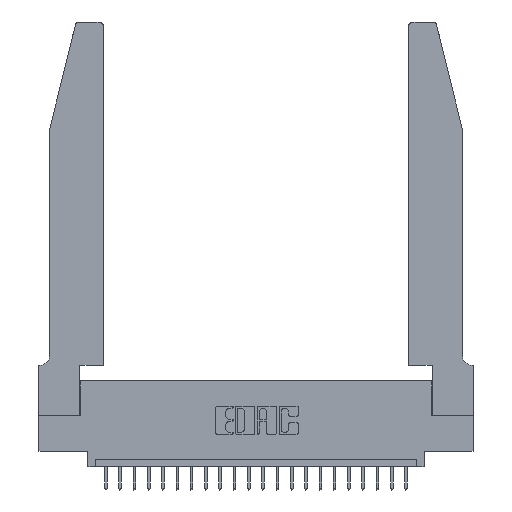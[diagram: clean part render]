
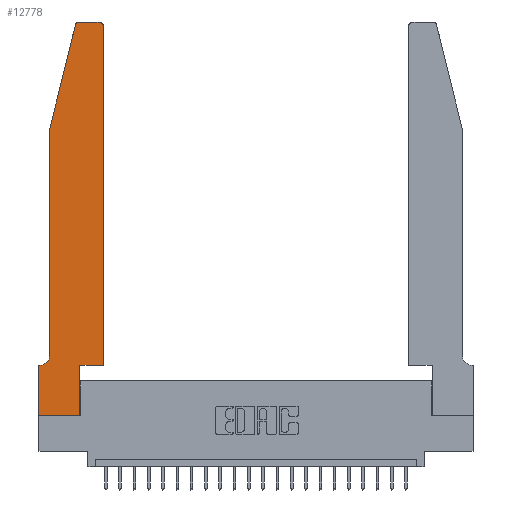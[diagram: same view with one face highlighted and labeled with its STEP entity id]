
A CAD part, top view. The second image highlights one B-rep face of the part: STEP entity #12778.
In plain terms, the highlighted planar face has unit normal (0, 0, 1).
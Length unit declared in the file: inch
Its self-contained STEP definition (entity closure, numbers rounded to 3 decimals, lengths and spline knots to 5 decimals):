
#12 = VERTEX_POINT ( 'NONE', #21400 ) ;
#245 = EDGE_CURVE ( 'NONE', #12, #11138, #21947, .T. ) ;
#420 = ORIENTED_EDGE ( 'NONE', *, *, #14623, .T. ) ;
#644 = DIRECTION ( 'NONE',  ( 1., 0., 0. ) ) ;
#722 = CARTESIAN_POINT ( 'NONE',  ( 0.4505, 0.35, 0.37 ) ) ;
#818 = VERTEX_POINT ( 'NONE', #722 ) ;
#968 = CARTESIAN_POINT ( 'NONE',  ( 0.0055, 0.35, 0.37 ) ) ;
#1003 = CARTESIAN_POINT ( 'NONE',  ( 0., 0.35, 0.37 ) ) ;
#1367 = LINE ( 'NONE', #20364, #1975 ) ;
#1441 = CARTESIAN_POINT ( 'NONE',  ( 0.4205, 2.72, 0.37 ) ) ;
#1541 = DIRECTION ( 'NONE',  ( 0., 0., -1. ) ) ;
#1650 = VERTEX_POINT ( 'NONE', #11311 ) ;
#1730 = VERTEX_POINT ( 'NONE', #23670 ) ;
#1876 = CARTESIAN_POINT ( 'NONE',  ( 0.2605, 2.75, 0.37 ) ) ;
#1975 = VECTOR ( 'NONE', #12963, 39.37008 ) ;
#2548 = ORIENTED_EDGE ( 'NONE', *, *, #4181, .T. ) ;
#2737 = CIRCLE ( 'NONE', #22688, 0.07 ) ;
#3608 = ORIENTED_EDGE ( 'NONE', *, *, #23975, .T. ) ;
#3681 = AXIS2_PLACEMENT_3D ( 'NONE', #12001, #17475, #15789 ) ;
#3734 = ORIENTED_EDGE ( 'NONE', *, *, #11519, .T. ) ;
#4095 = CIRCLE ( 'NONE', #3681, 0.03 ) ;
#4103 = VERTEX_POINT ( 'NONE', #8021 ) ;
#4181 = EDGE_CURVE ( 'NONE', #1730, #15587, #2737, .T. ) ;
#4785 = LINE ( 'NONE', #19580, #16541 ) ;
#5365 = VERTEX_POINT ( 'NONE', #7875 ) ;
#5584 = CARTESIAN_POINT ( 'NONE',  ( 0.4205, 2.75, 0.37 ) ) ;
#5873 = ORIENTED_EDGE ( 'NONE', *, *, #245, .T. ) ;
#5895 = EDGE_CURVE ( 'NONE', #5365, #20398, #1367, .T. ) ;
#6789 = EDGE_CURVE ( 'NONE', #20398, #1730, #19794, .T. ) ;
#7076 = DIRECTION ( 'NONE',  ( 1., 0., 0. ) ) ;
#7831 = EDGE_CURVE ( 'NONE', #15587, #19363, #4785, .T. ) ;
#7875 = CARTESIAN_POINT ( 'NONE',  ( 0.25487, 2.72718, 0.37 ) ) ;
#8021 = CARTESIAN_POINT ( 'NONE',  ( 0.2865, 0.35, 0.37 ) ) ;
#8172 = CARTESIAN_POINT ( 'NONE',  ( 0.4505, 0.35, 0.37 ) ) ;
#8364 = VECTOR ( 'NONE', #12646, 39.37008 ) ;
#8563 = CARTESIAN_POINT ( 'NONE',  ( 0.2865, 0., 0.37 ) ) ;
#8788 = ORIENTED_EDGE ( 'NONE', *, *, #6789, .T. ) ;
#8869 = VERTEX_POINT ( 'NONE', #21724 ) ;
#9479 = DIRECTION ( 'NONE',  ( 0., -1., 0. ) ) ;
#10090 = LINE ( 'NONE', #8172, #22071 ) ;
#10218 = LINE ( 'NONE', #1876, #18743 ) ;
#10506 = VECTOR ( 'NONE', #644, 39.37008 ) ;
#10783 = LINE ( 'NONE', #23120, #10506 ) ;
#10952 = DIRECTION ( 'NONE',  ( 0., 0., 1. ) ) ;
#11138 = VERTEX_POINT ( 'NONE', #8563 ) ;
#11145 = DIRECTION ( 'NONE',  ( -1., 0., 0. ) ) ;
#11148 = CARTESIAN_POINT ( 'NONE',  ( 0., 0., 0.37 ) ) ;
#11269 = DIRECTION ( 'NONE',  ( 1., 0., 0. ) ) ;
#11300 = DIRECTION ( 'NONE',  ( -1., 0., 0. ) ) ;
#11311 = CARTESIAN_POINT ( 'NONE',  ( 0.4505, 2.72, 0.37 ) ) ;
#11321 = AXIS2_PLACEMENT_3D ( 'NONE', #15298, #22427, #11269 ) ;
#11519 = EDGE_CURVE ( 'NONE', #16461, #8869, #10218, .T. ) ;
#11669 = EDGE_CURVE ( 'NONE', #4103, #818, #10783, .T. ) ;
#11670 = LINE ( 'NONE', #11148, #21845 ) ;
#12001 = CARTESIAN_POINT ( 'NONE',  ( 0.284, 2.72, 0.37 ) ) ;
#12327 = DIRECTION ( 'NONE',  ( -1., 0., 0. ) ) ;
#12646 = DIRECTION ( 'NONE',  ( 0., -1., 0. ) ) ;
#12778 = ADVANCED_FACE ( 'NONE', ( #16432 ), #17165, .T. ) ;
#12876 = CARTESIAN_POINT ( 'NONE',  ( 0., 0., 0.37 ) ) ;
#12921 = VECTOR ( 'NONE', #22213, 39.37008 ) ;
#12963 = DIRECTION ( 'NONE',  ( -0.239, -0.971, 0. ) ) ;
#14623 = EDGE_CURVE ( 'NONE', #19363, #12, #11670, .T. ) ;
#14729 = ORIENTED_EDGE ( 'NONE', *, *, #11669, .T. ) ;
#15298 = CARTESIAN_POINT ( 'NONE',  ( 0., 0.35, 0.37 ) ) ;
#15587 = VERTEX_POINT ( 'NONE', #968 ) ;
#15789 = DIRECTION ( 'NONE',  ( 1., 0., 0. ) ) ;
#15840 = DIRECTION ( 'NONE',  ( 0., 1., 0. ) ) ;
#16432 = FACE_OUTER_BOUND ( 'NONE', #24192, .T. ) ;
#16461 = VERTEX_POINT ( 'NONE', #5584 ) ;
#16541 = VECTOR ( 'NONE', #12327, 39.37008 ) ;
#16726 = CARTESIAN_POINT ( 'NONE',  ( 0.0055, 0.42, 0.37 ) ) ;
#17019 = EDGE_CURVE ( 'NONE', #818, #1650, #10090, .T. ) ;
#17165 = PLANE ( 'NONE',  #11321 ) ;
#17475 = DIRECTION ( 'NONE',  ( 0., 0., 1. ) ) ;
#17480 = ORIENTED_EDGE ( 'NONE', *, *, #5895, .T. ) ;
#17497 = ORIENTED_EDGE ( 'NONE', *, *, #19230, .T. ) ;
#18743 = VECTOR ( 'NONE', #11300, 39.37008 ) ;
#19230 = EDGE_CURVE ( 'NONE', #8869, #5365, #4095, .T. ) ;
#19363 = VERTEX_POINT ( 'NONE', #1003 ) ;
#19567 = ORIENTED_EDGE ( 'NONE', *, *, #17019, .T. ) ;
#19580 = CARTESIAN_POINT ( 'NONE',  ( 0.0755, 0.35, 0.37 ) ) ;
#19794 = LINE ( 'NONE', #21831, #8364 ) ;
#20082 = CARTESIAN_POINT ( 'NONE',  ( 0.2865, 0.35, 0.37 ) ) ;
#20364 = CARTESIAN_POINT ( 'NONE',  ( 0.0755, 2., 0.37 ) ) ;
#20398 = VERTEX_POINT ( 'NONE', #22776 ) ;
#20496 = ORIENTED_EDGE ( 'NONE', *, *, #7831, .T. ) ;
#20735 = EDGE_CURVE ( 'NONE', #11138, #4103, #23606, .T. ) ;
#21400 = CARTESIAN_POINT ( 'NONE',  ( 0., 0., 0.37 ) ) ;
#21574 = VECTOR ( 'NONE', #23569, 39.37008 ) ;
#21724 = CARTESIAN_POINT ( 'NONE',  ( 0.284, 2.75, 0.37 ) ) ;
#21831 = CARTESIAN_POINT ( 'NONE',  ( 0.0755, 2., 0.37 ) ) ;
#21845 = VECTOR ( 'NONE', #9479, 39.37008 ) ;
#21947 = LINE ( 'NONE', #12876, #12921 ) ;
#21982 = ORIENTED_EDGE ( 'NONE', *, *, #20735, .T. ) ;
#22071 = VECTOR ( 'NONE', #15840, 39.37008 ) ;
#22213 = DIRECTION ( 'NONE',  ( 1., 0., 0. ) ) ;
#22383 = AXIS2_PLACEMENT_3D ( 'NONE', #1441, #10952, #7076 ) ;
#22427 = DIRECTION ( 'NONE',  ( 0., 0., 1. ) ) ;
#22688 = AXIS2_PLACEMENT_3D ( 'NONE', #16726, #1541, #11145 ) ;
#22776 = CARTESIAN_POINT ( 'NONE',  ( 0.0755, 2., 0.37 ) ) ;
#23120 = CARTESIAN_POINT ( 'NONE',  ( 0.4505, 0.35, 0.37 ) ) ;
#23569 = DIRECTION ( 'NONE',  ( 0., 1., 0. ) ) ;
#23606 = LINE ( 'NONE', #20082, #21574 ) ;
#23670 = CARTESIAN_POINT ( 'NONE',  ( 0.0755, 0.42, 0.37 ) ) ;
#23975 = EDGE_CURVE ( 'NONE', #1650, #16461, #24015, .T. ) ;
#24015 = CIRCLE ( 'NONE', #22383, 0.03 ) ;
#24192 = EDGE_LOOP ( 'NONE', ( #3734, #17497, #17480, #8788, #2548, #20496, #420, #5873, #21982, #14729, #19567, #3608 ) ) ;
